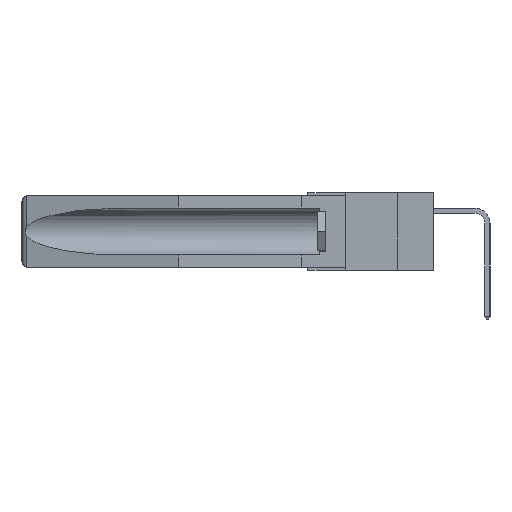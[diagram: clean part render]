
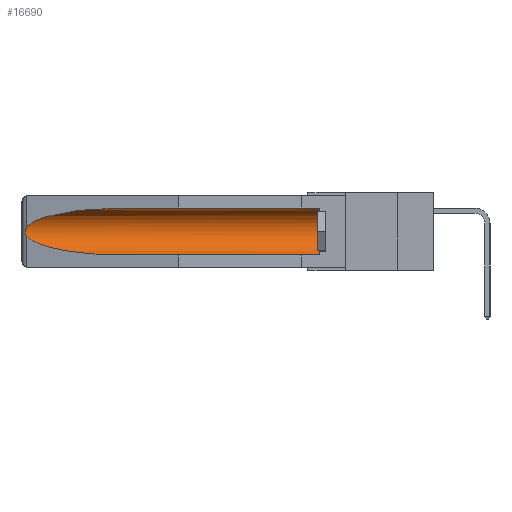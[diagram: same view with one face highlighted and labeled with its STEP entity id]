
A CAD part, left-side view. The second image highlights one B-rep face of the part: STEP entity #16690.
In plain terms, the highlighted cylindrical face has radius 2.857 mm (diameter 5.715 mm), a partial arc.
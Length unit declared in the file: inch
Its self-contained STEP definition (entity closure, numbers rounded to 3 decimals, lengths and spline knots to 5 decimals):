
#406 = CARTESIAN_POINT ( 'NONE',  ( 0.155, -0.30754, -0.1715 ) ) ;
#669 = CARTESIAN_POINT ( 'NONE',  ( 0.26597, 1.52961, -0.15275 ) ) ;
#965 =( BOUNDED_CURVE ( )  B_SPLINE_CURVE ( 3, ( #10600, #5660, #5439, #1730 ),
 .UNSPECIFIED., .F., .F. ) 
 B_SPLINE_CURVE_WITH_KNOTS ( ( 4, 4 ),
 ( 4.71239, 6.08839 ),
 .UNSPECIFIED. ) 
 CURVE ( )  GEOMETRIC_REPRESENTATION_ITEM ( )  RATIONAL_B_SPLINE_CURVE ( ( 1., 0.848, 0.848, 1. ) ) 
 REPRESENTATION_ITEM ( '' )  );
#1730 = CARTESIAN_POINT ( 'NONE',  ( 0.26537, 1.52718, -0.14972 ) ) ;
#2390 = VERTEX_POINT ( 'NONE', #9400 ) ;
#2652 = EDGE_CURVE ( 'NONE', #12600, #3593, #15560, .T. ) ;
#3170 = CARTESIAN_POINT ( 'NONE',  ( 0.26537, 1.52718, -0.14972 ) ) ;
#3233 = CARTESIAN_POINT ( 'NONE',  ( 0.26655, 1.53094, -0.18657 ) ) ;
#3390 = CARTESIAN_POINT ( 'NONE',  ( 0.26537, 1.52718, -0.19328 ) ) ;
#3459 = VECTOR ( 'NONE', #15181, 39.37008 ) ;
#3593 = VERTEX_POINT ( 'NONE', #5752 ) ;
#4037 = LINE ( 'NONE', #15874, #3459 ) ;
#4432 = EDGE_CURVE ( 'NONE', #12600, #8904, #14025, .T. ) ;
#4996 = CARTESIAN_POINT ( 'NONE',  ( 0.155, 0.126, -0.059 ) ) ;
#5310 = CARTESIAN_POINT ( 'NONE',  ( 0.26537, 1.52718, -0.19328 ) ) ;
#5375 = CYLINDRICAL_SURFACE ( 'NONE', #13727, 0.1125 ) ;
#5439 = CARTESIAN_POINT ( 'NONE',  ( 0.25451, 1.48313, -0.09465 ) ) ;
#5660 = CARTESIAN_POINT ( 'NONE',  ( 0.21114, 1.30732, -0.059 ) ) ;
#5724 = VERTEX_POINT ( 'NONE', #15364 ) ;
#5752 = CARTESIAN_POINT ( 'NONE',  ( 0.155, 1.07973, -0.284 ) ) ;
#5755 = DIRECTION ( 'NONE',  ( 0., 1., 0. ) ) ;
#5806 = VERTEX_POINT ( 'NONE', #5310 ) ;
#6893 = EDGE_CURVE ( 'NONE', #5724, #2390, #965, .T. ) ;
#7276 = DIRECTION ( 'NONE',  ( 0., -1., 0. ) ) ;
#7286 = CARTESIAN_POINT ( 'NONE',  ( 0.155, 1.07973, -0.284 ) ) ;
#7388 = DIRECTION ( 'NONE',  ( 0., 0., 1. ) ) ;
#7522 = EDGE_CURVE ( 'NONE', #2390, #5806, #15021, .T. ) ;
#8601 = CARTESIAN_POINT ( 'NONE',  ( 0.21114, 1.30732, -0.284 ) ) ;
#8904 = VERTEX_POINT ( 'NONE', #4996 ) ;
#9400 = CARTESIAN_POINT ( 'NONE',  ( 0.26537, 1.52718, -0.14972 ) ) ;
#9692 = CARTESIAN_POINT ( 'NONE',  ( 0.2673, 1.5327, -0.16383 ) ) ;
#10408 = FACE_OUTER_BOUND ( 'NONE', #15323, .T. ) ;
#10560 = AXIS2_PLACEMENT_3D ( 'NONE', #16553, #7276, #7388 ) ;
#10586 = CARTESIAN_POINT ( 'NONE',  ( 0.26537, 1.52718, -0.19328 ) ) ;
#10600 = CARTESIAN_POINT ( 'NONE',  ( 0.155, 1.07973, -0.059 ) ) ;
#10962 = CARTESIAN_POINT ( 'NONE',  ( 0.26597, 1.5296, -0.19026 ) ) ;
#11028 = CARTESIAN_POINT ( 'NONE',  ( 0.2675, 1.53308, -0.16763 ) ) ;
#11466 = ORIENTED_EDGE ( 'NONE', *, *, #12971, .T. ) ;
#12110 = VECTOR ( 'NONE', #16449, 39.37008 ) ;
#12221 = CARTESIAN_POINT ( 'NONE',  ( 0.2675, 1.53308, -0.17534 ) ) ;
#12600 = VERTEX_POINT ( 'NONE', #13438 ) ;
#12806 =( BOUNDED_CURVE ( )  B_SPLINE_CURVE ( 3, ( #10586, #14492, #8601, #7286 ),
 .UNSPECIFIED., .F., .F. ) 
 B_SPLINE_CURVE_WITH_KNOTS ( ( 4, 4 ),
 ( 0.1948, 1.5708 ),
 .UNSPECIFIED. ) 
 CURVE ( )  GEOMETRIC_REPRESENTATION_ITEM ( )  RATIONAL_B_SPLINE_CURVE ( ( 1., 0.848, 0.848, 1. ) ) 
 REPRESENTATION_ITEM ( '' )  );
#12959 = ORIENTED_EDGE ( 'NONE', *, *, #13542, .T. ) ;
#12971 = EDGE_CURVE ( 'NONE', #5806, #3593, #12806, .T. ) ;
#13438 = CARTESIAN_POINT ( 'NONE',  ( 0.155, 0.126, -0.284 ) ) ;
#13472 = CARTESIAN_POINT ( 'NONE',  ( 0.26654, 1.53092, -0.15636 ) ) ;
#13542 = EDGE_CURVE ( 'NONE', #8904, #5724, #4037, .T. ) ;
#13727 = AXIS2_PLACEMENT_3D ( 'NONE', #406, #5755, #15979 ) ;
#14025 = CIRCLE ( 'NONE', #10560, 0.1125 ) ;
#14492 = CARTESIAN_POINT ( 'NONE',  ( 0.25451, 1.48313, -0.24835 ) ) ;
#15021 = B_SPLINE_CURVE_WITH_KNOTS ( 'NONE', 3,
 ( #3170, #669, #13472, #9692, #11028, #12221, #16192, #3233, #10962, #3390 ),
 .UNSPECIFIED., .F., .F.,
 ( 4, 2, 2, 2, 4 ),
 ( 0., 0.00029, 0.00058, 0.00087, 0.00117 ),
 .UNSPECIFIED. ) ;
#15181 = DIRECTION ( 'NONE',  ( 0., 1., 0. ) ) ;
#15323 = EDGE_LOOP ( 'NONE', ( #16095, #16297, #11466, #16320, #16326, #12959 ) ) ;
#15364 = CARTESIAN_POINT ( 'NONE',  ( 0.155, 1.07973, -0.059 ) ) ;
#15560 = LINE ( 'NONE', #16505, #12110 ) ;
#15874 = CARTESIAN_POINT ( 'NONE',  ( 0.155, -0.30754, -0.059 ) ) ;
#15979 = DIRECTION ( 'NONE',  ( 0., 0., 1. ) ) ;
#16095 = ORIENTED_EDGE ( 'NONE', *, *, #6893, .T. ) ;
#16192 = CARTESIAN_POINT ( 'NONE',  ( 0.2673, 1.53269, -0.17917 ) ) ;
#16297 = ORIENTED_EDGE ( 'NONE', *, *, #7522, .T. ) ;
#16320 = ORIENTED_EDGE ( 'NONE', *, *, #2652, .F. ) ;
#16326 = ORIENTED_EDGE ( 'NONE', *, *, #4432, .T. ) ;
#16449 = DIRECTION ( 'NONE',  ( 0., 1., 0. ) ) ;
#16505 = CARTESIAN_POINT ( 'NONE',  ( 0.155, -0.30754, -0.284 ) ) ;
#16553 = CARTESIAN_POINT ( 'NONE',  ( 0.155, 0.126, -0.1715 ) ) ;
#16690 = ADVANCED_FACE ( 'NONE', ( #10408 ), #5375, .F. ) ;
